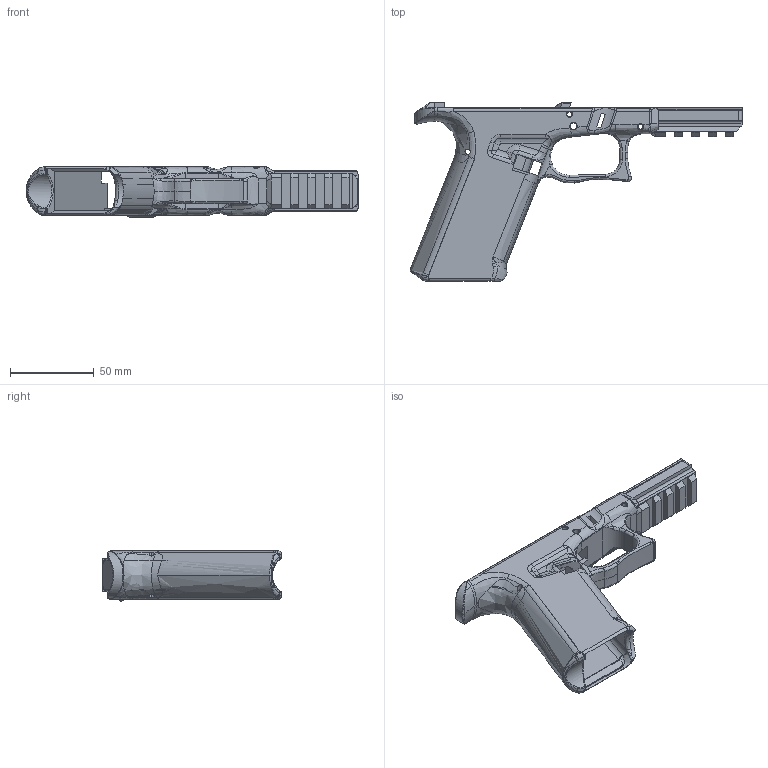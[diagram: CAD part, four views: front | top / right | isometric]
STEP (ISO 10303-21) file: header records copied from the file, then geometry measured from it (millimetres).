
FILE_DESCRIPTION (( 'STEP AP214' ), '1' );
FILE_NAME ('FMDA DD17.2 BTPR.STEP', '2022-03-03T17:59:38', ( '' ), ( '' ), 'SwSTEP 2.0', 'SolidWorks 2021', '' );
FILE_SCHEMA (( 'AUTOMOTIVE_DESIGN' ));
Length unit declared in the file: millimetre
Products named in the file (1): FMDA DD17.2 BTPR
Bounding box: 197.63 x 106.5 x 29.84 mm (x, y, z)
Volume: 87135.8 mm3; surface area: 48484.9 mm2
Topology: 1 solids, 1 shells, 804 faces, 2240 edges, 1410 vertices
Faces by surface type: bspline 312, cylinder 217, plane 202, torus 33, sphere 26, cone 14
Entity records: 52229 total; most frequent: CARTESIAN_POINT 34558, ORIENTED_EDGE 4462, DIRECTION 2625, EDGE_CURVE 2231, VERTEX_POINT 1410, AXIS2_PLACEMENT_3D 899, B_SPLINE_CURVE_WITH_KNOTS 861, LINE 827
